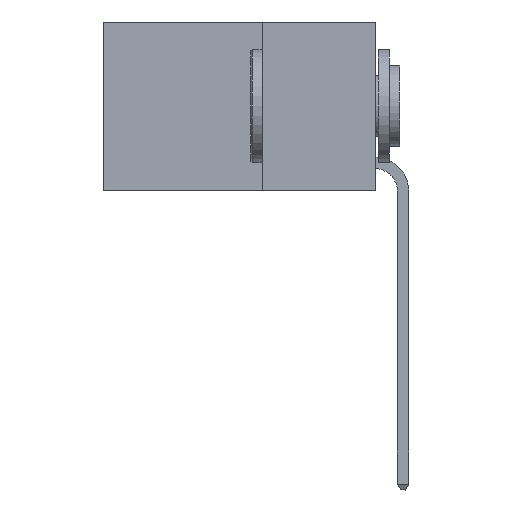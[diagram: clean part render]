
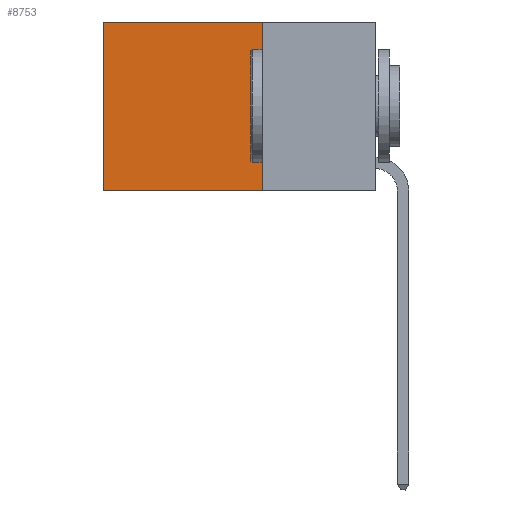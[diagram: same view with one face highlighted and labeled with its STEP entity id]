
A CAD part, left-side view. The second image highlights one B-rep face of the part: STEP entity #8753.
In plain terms, the highlighted planar face has unit normal (-1, 0, 0).
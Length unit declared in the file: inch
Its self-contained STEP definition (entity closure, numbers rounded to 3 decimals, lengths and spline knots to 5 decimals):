
#393 = VERTEX_POINT ( 'NONE', #1137 ) ;
#794 = AXIS2_PLACEMENT_3D ( 'NONE', #26567, #14217, #1780 ) ;
#1137 = CARTESIAN_POINT ( 'NONE',  ( 0.2625, 0.6, 0. ) ) ;
#1780 = DIRECTION ( 'NONE',  ( 0., 0., -1. ) ) ;
#2062 = CARTESIAN_POINT ( 'NONE',  ( 0.2625, 0.25, 0. ) ) ;
#2392 = ORIENTED_EDGE ( 'NONE', *, *, #26639, .F. ) ;
#3018 = CARTESIAN_POINT ( 'NONE',  ( 0.2625, 0.6, -0.37 ) ) ;
#3172 = VECTOR ( 'NONE', #5632, 39.37008 ) ;
#3795 = LINE ( 'NONE', #8456, #25136 ) ;
#4285 = DIRECTION ( 'NONE',  ( 0., 1., 0. ) ) ;
#4553 = CARTESIAN_POINT ( 'NONE',  ( 0.2625, 0.25, -0.37 ) ) ;
#5313 = VECTOR ( 'NONE', #22700, 39.37008 ) ;
#5632 = DIRECTION ( 'NONE',  ( 0., 1., 0. ) ) ;
#8456 = CARTESIAN_POINT ( 'NONE',  ( 0.2625, 0.25, -0.37 ) ) ;
#8753 = ADVANCED_FACE ( 'NONE', ( #19662 ), #10070, .F. ) ;
#9507 = DIRECTION ( 'NONE',  ( 0., 0., -1. ) ) ;
#10070 = PLANE ( 'NONE',  #794 ) ;
#10739 = EDGE_CURVE ( 'NONE', #10781, #10842, #25986, .T. ) ;
#10781 = VERTEX_POINT ( 'NONE', #22888 ) ;
#10842 = VERTEX_POINT ( 'NONE', #4553 ) ;
#13516 = LINE ( 'NONE', #23940, #23848 ) ;
#14217 = DIRECTION ( 'NONE',  ( 1., 0., 0. ) ) ;
#19662 = FACE_OUTER_BOUND ( 'NONE', #24036, .T. ) ;
#19668 = ORIENTED_EDGE ( 'NONE', *, *, #10739, .F. ) ;
#20052 = VERTEX_POINT ( 'NONE', #3018 ) ;
#22335 = EDGE_CURVE ( 'NONE', #10781, #393, #25165, .T. ) ;
#22700 = DIRECTION ( 'NONE',  ( 0., 0., -1. ) ) ;
#22806 = EDGE_CURVE ( 'NONE', #393, #20052, #13516, .T. ) ;
#22888 = CARTESIAN_POINT ( 'NONE',  ( 0.2625, 0.25, 0. ) ) ;
#23011 = ORIENTED_EDGE ( 'NONE', *, *, #22335, .T. ) ;
#23848 = VECTOR ( 'NONE', #9507, 39.37008 ) ;
#23940 = CARTESIAN_POINT ( 'NONE',  ( 0.2625, 0.6, 0. ) ) ;
#24036 = EDGE_LOOP ( 'NONE', ( #25162, #2392, #19668, #23011 ) ) ;
#25136 = VECTOR ( 'NONE', #4285, 39.37008 ) ;
#25162 = ORIENTED_EDGE ( 'NONE', *, *, #22806, .T. ) ;
#25165 = LINE ( 'NONE', #26212, #3172 ) ;
#25986 = LINE ( 'NONE', #2062, #5313 ) ;
#26212 = CARTESIAN_POINT ( 'NONE',  ( 0.2625, 0.25, 0. ) ) ;
#26567 = CARTESIAN_POINT ( 'NONE',  ( 0.2625, 0.25, 0. ) ) ;
#26639 = EDGE_CURVE ( 'NONE', #10842, #20052, #3795, .T. ) ;
